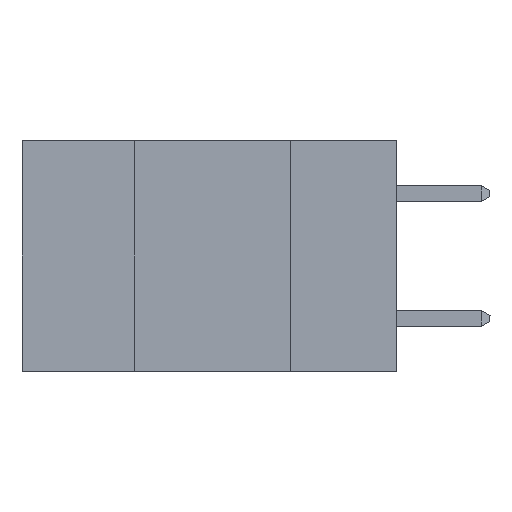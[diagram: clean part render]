
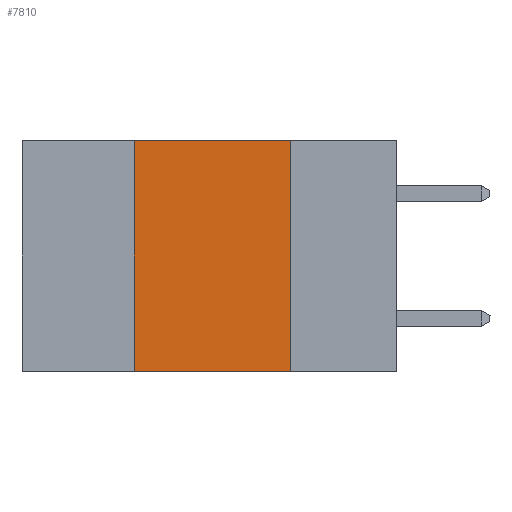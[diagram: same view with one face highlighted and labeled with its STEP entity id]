
A CAD part, left-side view. The second image highlights one B-rep face of the part: STEP entity #7810.
In plain terms, the highlighted planar face has unit normal (-1, 0, 0).
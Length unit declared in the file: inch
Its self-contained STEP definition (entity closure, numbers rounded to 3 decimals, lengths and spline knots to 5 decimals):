
#27 = VERTEX_POINT ( 'NONE', #1599 ) ;
#76 = DIRECTION ( 'NONE',  ( 1., 0., 0. ) ) ;
#581 = ORIENTED_EDGE ( 'NONE', *, *, #3755, .F. ) ;
#1039 = DIRECTION ( 'NONE',  ( 0., 0., -1. ) ) ;
#1087 = DIRECTION ( 'NONE',  ( 0., -1., 0. ) ) ;
#1569 = FACE_OUTER_BOUND ( 'NONE', #11602, .T. ) ;
#1599 = CARTESIAN_POINT ( 'NONE',  ( 0., 0.17, 0. ) ) ;
#1748 = ORIENTED_EDGE ( 'NONE', *, *, #10032, .T. ) ;
#1852 = VECTOR ( 'NONE', #7543, 39.37008 ) ;
#1938 = LINE ( 'NONE', #8842, #3763 ) ;
#1971 = DIRECTION ( 'NONE',  ( 0., 0., 1. ) ) ;
#2129 = CARTESIAN_POINT ( 'NONE',  ( 0., 0.6, 0. ) ) ;
#2312 = CARTESIAN_POINT ( 'NONE',  ( 0., 0.42, 0. ) ) ;
#2846 = CARTESIAN_POINT ( 'NONE',  ( 0., 0.17, 0. ) ) ;
#3755 = EDGE_CURVE ( 'NONE', #5969, #9391, #1938, .T. ) ;
#3763 = VECTOR ( 'NONE', #1971, 39.37008 ) ;
#4443 = VECTOR ( 'NONE', #1087, 39.37008 ) ;
#5628 = VECTOR ( 'NONE', #8962, 39.37008 ) ;
#5652 = LINE ( 'NONE', #2846, #1852 ) ;
#5689 = LINE ( 'NONE', #2129, #4443 ) ;
#5969 = VERTEX_POINT ( 'NONE', #12581 ) ;
#6022 = ORIENTED_EDGE ( 'NONE', *, *, #9060, .F. ) ;
#7495 = ORIENTED_EDGE ( 'NONE', *, *, #12465, .F. ) ;
#7543 = DIRECTION ( 'NONE',  ( 0., 0., -1. ) ) ;
#7810 = ADVANCED_FACE ( 'NONE', ( #1569 ), #7943, .F. ) ;
#7943 = PLANE ( 'NONE',  #10919 ) ;
#7989 = CARTESIAN_POINT ( 'NONE',  ( 0., 0.6, -0.37 ) ) ;
#8762 = CARTESIAN_POINT ( 'NONE',  ( 0., 0.17, -0.37 ) ) ;
#8787 = LINE ( 'NONE', #7989, #5628 ) ;
#8842 = CARTESIAN_POINT ( 'NONE',  ( 0., 0.42, 0. ) ) ;
#8962 = DIRECTION ( 'NONE',  ( 0., -1., 0. ) ) ;
#9060 = EDGE_CURVE ( 'NONE', #27, #9304, #5652, .T. ) ;
#9304 = VERTEX_POINT ( 'NONE', #8762 ) ;
#9391 = VERTEX_POINT ( 'NONE', #2312 ) ;
#10032 = EDGE_CURVE ( 'NONE', #5969, #9304, #8787, .T. ) ;
#10919 = AXIS2_PLACEMENT_3D ( 'NONE', #10921, #76, #1039 ) ;
#10921 = CARTESIAN_POINT ( 'NONE',  ( 0., 0.6, 0. ) ) ;
#11602 = EDGE_LOOP ( 'NONE', ( #6022, #7495, #581, #1748 ) ) ;
#12465 = EDGE_CURVE ( 'NONE', #9391, #27, #5689, .T. ) ;
#12581 = CARTESIAN_POINT ( 'NONE',  ( 0., 0.42, -0.37 ) ) ;
